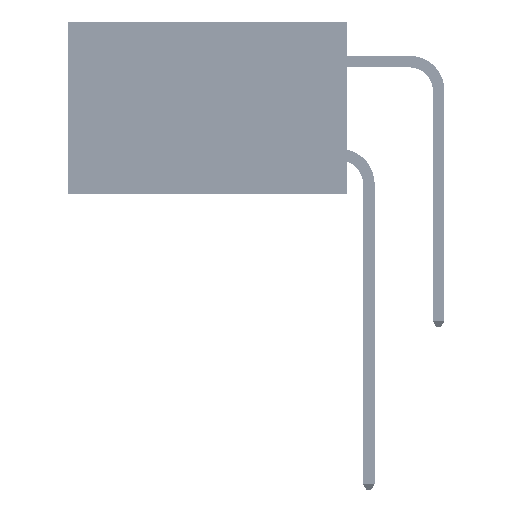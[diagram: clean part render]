
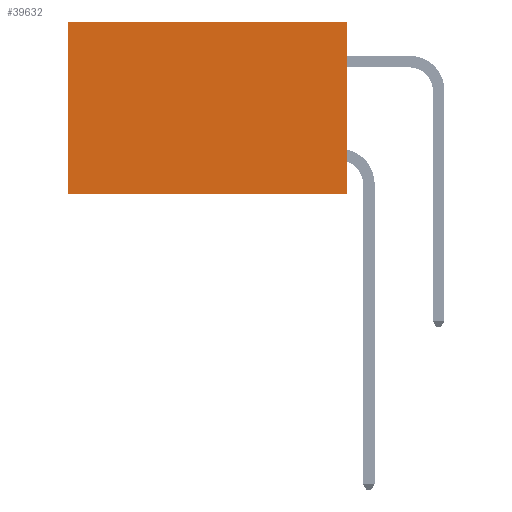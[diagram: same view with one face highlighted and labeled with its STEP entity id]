
A CAD part, left-side view. The second image highlights one B-rep face of the part: STEP entity #39632.
In plain terms, the highlighted planar face has unit normal (-1, 0, 0).
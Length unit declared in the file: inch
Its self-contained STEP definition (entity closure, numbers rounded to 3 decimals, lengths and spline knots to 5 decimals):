
#1631 = CARTESIAN_POINT ( 'NONE',  ( 0.2875, 0.6, 0. ) ) ;
#3496 = VERTEX_POINT ( 'NONE', #40122 ) ;
#3567 = CARTESIAN_POINT ( 'NONE',  ( 0.2875, 0., 0. ) ) ;
#5737 = DIRECTION ( 'NONE',  ( 0., 1., 0. ) ) ;
#6847 = AXIS2_PLACEMENT_3D ( 'NONE', #3567, #39500, #8079 ) ;
#7273 = LINE ( 'NONE', #1631, #36875 ) ;
#8079 = DIRECTION ( 'NONE',  ( 0., 0., -1. ) ) ;
#8460 = VECTOR ( 'NONE', #5737, 39.37008 ) ;
#9888 = DIRECTION ( 'NONE',  ( 0., 0., -1. ) ) ;
#11211 = CARTESIAN_POINT ( 'NONE',  ( 0.2875, 0., 0. ) ) ;
#12198 = CARTESIAN_POINT ( 'NONE',  ( 0.2875, 0.6, -0.37 ) ) ;
#13331 = CARTESIAN_POINT ( 'NONE',  ( 0.2875, 0., -0.37 ) ) ;
#15388 = EDGE_CURVE ( 'NONE', #35914, #33882, #39302, .T. ) ;
#16944 = ORIENTED_EDGE ( 'NONE', *, *, #15388, .F. ) ;
#17592 = VECTOR ( 'NONE', #40881, 39.37008 ) ;
#19544 = ORIENTED_EDGE ( 'NONE', *, *, #20131, .T. ) ;
#20131 = EDGE_CURVE ( 'NONE', #3496, #33320, #26635, .T. ) ;
#20741 = ORIENTED_EDGE ( 'NONE', *, *, #43107, .F. ) ;
#22888 = FACE_OUTER_BOUND ( 'NONE', #29966, .T. ) ;
#22929 = ORIENTED_EDGE ( 'NONE', *, *, #38488, .T. ) ;
#26552 = PLANE ( 'NONE',  #6847 ) ;
#26635 = LINE ( 'NONE', #40368, #8460 ) ;
#28669 = CARTESIAN_POINT ( 'NONE',  ( 0.2875, 0.6, 0. ) ) ;
#29966 = EDGE_LOOP ( 'NONE', ( #22929, #16944, #20741, #19544 ) ) ;
#33320 = VERTEX_POINT ( 'NONE', #28669 ) ;
#33882 = VERTEX_POINT ( 'NONE', #12198 ) ;
#35914 = VERTEX_POINT ( 'NONE', #47795 ) ;
#36875 = VECTOR ( 'NONE', #9888, 39.37008 ) ;
#38142 = VECTOR ( 'NONE', #38225, 39.37008 ) ;
#38225 = DIRECTION ( 'NONE',  ( 0., 0., -1. ) ) ;
#38488 = EDGE_CURVE ( 'NONE', #33320, #33882, #7273, .T. ) ;
#39302 = LINE ( 'NONE', #13331, #17592 ) ;
#39500 = DIRECTION ( 'NONE',  ( 1., 0., 0. ) ) ;
#39632 = ADVANCED_FACE ( 'NONE', ( #22888 ), #26552, .F. ) ;
#39938 = LINE ( 'NONE', #11211, #38142 ) ;
#40122 = CARTESIAN_POINT ( 'NONE',  ( 0.2875, 0., 0. ) ) ;
#40368 = CARTESIAN_POINT ( 'NONE',  ( 0.2875, 0., 0. ) ) ;
#40881 = DIRECTION ( 'NONE',  ( 0., 1., 0. ) ) ;
#43107 = EDGE_CURVE ( 'NONE', #3496, #35914, #39938, .T. ) ;
#47795 = CARTESIAN_POINT ( 'NONE',  ( 0.2875, 0., -0.37 ) ) ;
